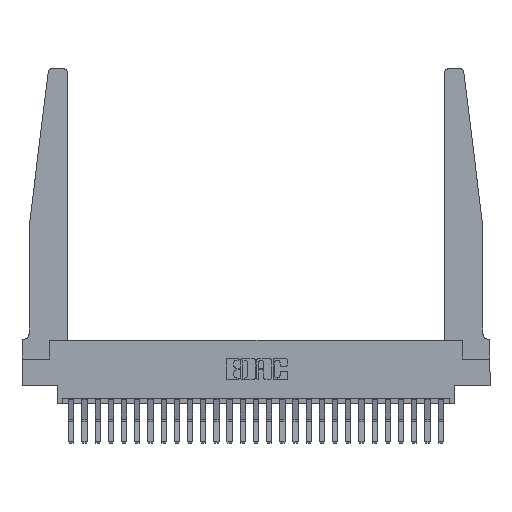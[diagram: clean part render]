
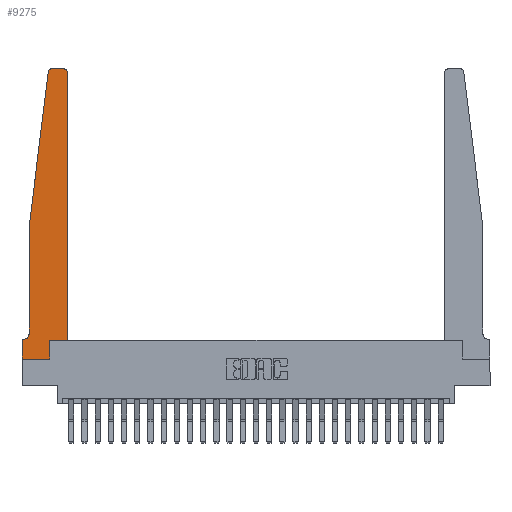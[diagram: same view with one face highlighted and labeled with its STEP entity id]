
A CAD part, top view. The second image highlights one B-rep face of the part: STEP entity #9275.
In plain terms, the highlighted planar face has unit normal (0, 0, 1).
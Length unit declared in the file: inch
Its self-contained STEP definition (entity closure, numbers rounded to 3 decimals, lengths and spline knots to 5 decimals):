
#525 = CARTESIAN_POINT ( 'NONE',  ( 0.27653, 2.75, 0.37 ) ) ;
#551 = LINE ( 'NONE', #2809, #6675 ) ;
#752 = DIRECTION ( 'NONE',  ( -1., 0., 0. ) ) ;
#1171 = DIRECTION ( 'NONE',  ( -1., 0., 0. ) ) ;
#1662 = AXIS2_PLACEMENT_3D ( 'NONE', #2229, #10287, #752 ) ;
#2229 = CARTESIAN_POINT ( 'NONE',  ( 0.015, 0.2375, 0.37 ) ) ;
#2302 = ORIENTED_EDGE ( 'NONE', *, *, #5409, .T. ) ;
#2438 = ORIENTED_EDGE ( 'NONE', *, *, #13744, .T. ) ;
#2572 = EDGE_CURVE ( 'NONE', #4891, #22221, #15211, .T. ) ;
#2788 = EDGE_CURVE ( 'NONE', #22221, #14991, #15902, .T. ) ;
#2809 = CARTESIAN_POINT ( 'NONE',  ( 0.2605, 0.18, 0.37 ) ) ;
#2926 = FACE_OUTER_BOUND ( 'NONE', #24799, .T. ) ;
#2995 = CARTESIAN_POINT ( 'NONE',  ( 0.2605, 0., 0.37 ) ) ;
#3048 = CARTESIAN_POINT ( 'NONE',  ( 0., 0.1875, 0.37 ) ) ;
#3547 = VECTOR ( 'NONE', #18163, 39.37008 ) ;
#3763 = DIRECTION ( 'NONE',  ( 0., 1., 0. ) ) ;
#3927 = CARTESIAN_POINT ( 'NONE',  ( 0.065, 0.2375, 0.37 ) ) ;
#4667 = CARTESIAN_POINT ( 'NONE',  ( 0.27653, 2.72, 0.37 ) ) ;
#4761 = EDGE_CURVE ( 'NONE', #23351, #17862, #11696, .T. ) ;
#4891 = VERTEX_POINT ( 'NONE', #18184 ) ;
#5033 = DIRECTION ( 'NONE',  ( 1., 0., 0. ) ) ;
#5409 = EDGE_CURVE ( 'NONE', #11388, #22050, #551, .T. ) ;
#5750 = AXIS2_PLACEMENT_3D ( 'NONE', #3048, #23415, #5033 ) ;
#5881 = VERTEX_POINT ( 'NONE', #14610 ) ;
#6675 = VECTOR ( 'NONE', #16571, 39.37008 ) ;
#6862 = VERTEX_POINT ( 'NONE', #525 ) ;
#7108 = DIRECTION ( 'NONE',  ( -1., 0., 0. ) ) ;
#7112 = EDGE_CURVE ( 'NONE', #5881, #6862, #13482, .T. ) ;
#7468 = DIRECTION ( 'NONE',  ( 0., -1., 0. ) ) ;
#7698 = CARTESIAN_POINT ( 'NONE',  ( 0.425, 2.72, 0.37 ) ) ;
#7784 = VECTOR ( 'NONE', #1171, 39.37008 ) ;
#8197 = ORIENTED_EDGE ( 'NONE', *, *, #2788, .T. ) ;
#8600 = CARTESIAN_POINT ( 'NONE',  ( 0.2605, 0.18, 0.37 ) ) ;
#8799 = EDGE_CURVE ( 'NONE', #14991, #11306, #15426, .T. ) ;
#9191 = LINE ( 'NONE', #13439, #19008 ) ;
#9195 = DIRECTION ( 'NONE',  ( 1., 0., 0. ) ) ;
#9275 = ADVANCED_FACE ( 'NONE', ( #2926 ), #19318, .T. ) ;
#9444 = ORIENTED_EDGE ( 'NONE', *, *, #24372, .T. ) ;
#9576 = AXIS2_PLACEMENT_3D ( 'NONE', #4667, #14720, #12605 ) ;
#9729 = EDGE_CURVE ( 'NONE', #17698, #4891, #24715, .T. ) ;
#9831 = CARTESIAN_POINT ( 'NONE',  ( 0.425, 0.18, 0.37 ) ) ;
#10259 = EDGE_CURVE ( 'NONE', #11306, #23062, #9191, .T. ) ;
#10287 = DIRECTION ( 'NONE',  ( 0., 0., -1. ) ) ;
#11306 = VERTEX_POINT ( 'NONE', #18877 ) ;
#11388 = VERTEX_POINT ( 'NONE', #2995 ) ;
#11696 = LINE ( 'NONE', #9831, #21759 ) ;
#12215 = CARTESIAN_POINT ( 'NONE',  ( 0.015, 0.1875, 0.37 ) ) ;
#12524 = ORIENTED_EDGE ( 'NONE', *, *, #4761, .T. ) ;
#12605 = DIRECTION ( 'NONE',  ( 1., 0., 0. ) ) ;
#13300 = CARTESIAN_POINT ( 'NONE',  ( 0.395, 2.72, 0.37 ) ) ;
#13303 = ORIENTED_EDGE ( 'NONE', *, *, #2572, .T. ) ;
#13317 = CARTESIAN_POINT ( 'NONE',  ( 0.065, 0.1875, 0.37 ) ) ;
#13439 = CARTESIAN_POINT ( 'NONE',  ( 0., 0., 0.37 ) ) ;
#13482 = LINE ( 'NONE', #17573, #7784 ) ;
#13744 = EDGE_CURVE ( 'NONE', #6862, #17698, #25610, .T. ) ;
#14610 = CARTESIAN_POINT ( 'NONE',  ( 0.395, 2.75, 0.37 ) ) ;
#14720 = DIRECTION ( 'NONE',  ( 0., 0., 1. ) ) ;
#14762 = VECTOR ( 'NONE', #25852, 39.37008 ) ;
#14879 = CARTESIAN_POINT ( 'NONE',  ( 0.24675, 2.72367, 0.37 ) ) ;
#14959 = VECTOR ( 'NONE', #19024, 39.37008 ) ;
#14991 = VERTEX_POINT ( 'NONE', #12215 ) ;
#15211 = LINE ( 'NONE', #23289, #23566 ) ;
#15426 = LINE ( 'NONE', #13317, #18243 ) ;
#15427 = ORIENTED_EDGE ( 'NONE', *, *, #7112, .T. ) ;
#15902 = CIRCLE ( 'NONE', #1662, 0.05 ) ;
#16140 = EDGE_CURVE ( 'NONE', #23062, #11388, #22037, .T. ) ;
#16571 = DIRECTION ( 'NONE',  ( 0., 1., 0. ) ) ;
#16889 = DIRECTION ( 'NONE',  ( 0., 0., 1. ) ) ;
#17124 = CARTESIAN_POINT ( 'NONE',  ( 0., 0., 0.37 ) ) ;
#17573 = CARTESIAN_POINT ( 'NONE',  ( 0.25, 2.75, 0.37 ) ) ;
#17698 = VERTEX_POINT ( 'NONE', #14879 ) ;
#17862 = VERTEX_POINT ( 'NONE', #7698 ) ;
#18163 = DIRECTION ( 'NONE',  ( 1., 0., 0. ) ) ;
#18184 = CARTESIAN_POINT ( 'NONE',  ( 0.065, 1.25, 0.37 ) ) ;
#18243 = VECTOR ( 'NONE', #7108, 39.37008 ) ;
#18877 = CARTESIAN_POINT ( 'NONE',  ( 0., 0.1875, 0.37 ) ) ;
#19008 = VECTOR ( 'NONE', #7468, 39.37008 ) ;
#19024 = DIRECTION ( 'NONE',  ( -0.122, -0.992, 0. ) ) ;
#19318 = PLANE ( 'NONE',  #5750 ) ;
#20346 = ORIENTED_EDGE ( 'NONE', *, *, #9729, .T. ) ;
#20508 = ORIENTED_EDGE ( 'NONE', *, *, #22452, .T. ) ;
#20536 = CARTESIAN_POINT ( 'NONE',  ( 0., 0., 0.37 ) ) ;
#20899 = CARTESIAN_POINT ( 'NONE',  ( 0.425, 0.18, 0.37 ) ) ;
#21213 = AXIS2_PLACEMENT_3D ( 'NONE', #13300, #16889, #9195 ) ;
#21759 = VECTOR ( 'NONE', #3763, 39.37008 ) ;
#22037 = LINE ( 'NONE', #17124, #14762 ) ;
#22050 = VERTEX_POINT ( 'NONE', #8600 ) ;
#22092 = ORIENTED_EDGE ( 'NONE', *, *, #8799, .T. ) ;
#22221 = VERTEX_POINT ( 'NONE', #3927 ) ;
#22388 = LINE ( 'NONE', #22640, #3547 ) ;
#22452 = EDGE_CURVE ( 'NONE', #17862, #5881, #22928, .T. ) ;
#22640 = CARTESIAN_POINT ( 'NONE',  ( 0.425, 0.18, 0.37 ) ) ;
#22928 = CIRCLE ( 'NONE', #21213, 0.03 ) ;
#23062 = VERTEX_POINT ( 'NONE', #20536 ) ;
#23250 = ORIENTED_EDGE ( 'NONE', *, *, #10259, .T. ) ;
#23289 = CARTESIAN_POINT ( 'NONE',  ( 0.065, 1.25, 0.37 ) ) ;
#23351 = VERTEX_POINT ( 'NONE', #20899 ) ;
#23415 = DIRECTION ( 'NONE',  ( 0., 0., 1. ) ) ;
#23566 = VECTOR ( 'NONE', #25493, 39.37008 ) ;
#24372 = EDGE_CURVE ( 'NONE', #22050, #23351, #22388, .T. ) ;
#24588 = ORIENTED_EDGE ( 'NONE', *, *, #16140, .T. ) ;
#24715 = LINE ( 'NONE', #24957, #14959 ) ;
#24799 = EDGE_LOOP ( 'NONE', ( #15427, #2438, #20346, #13303, #8197, #22092, #23250, #24588, #2302, #9444, #12524, #20508 ) ) ;
#24957 = CARTESIAN_POINT ( 'NONE',  ( 0.065, 1.25, 0.37 ) ) ;
#25493 = DIRECTION ( 'NONE',  ( 0., -1., 0. ) ) ;
#25610 = CIRCLE ( 'NONE', #9576, 0.03 ) ;
#25852 = DIRECTION ( 'NONE',  ( 1., 0., 0. ) ) ;
